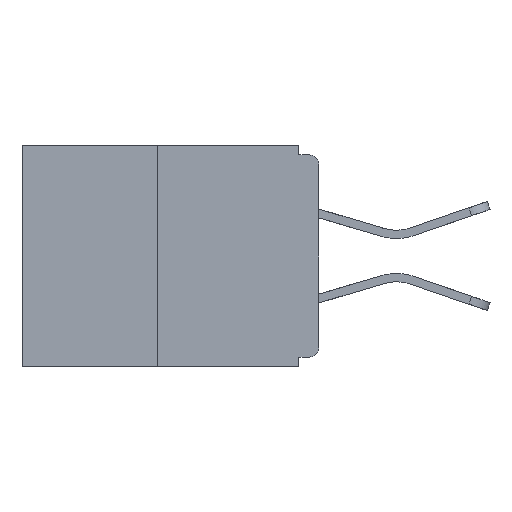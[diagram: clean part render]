
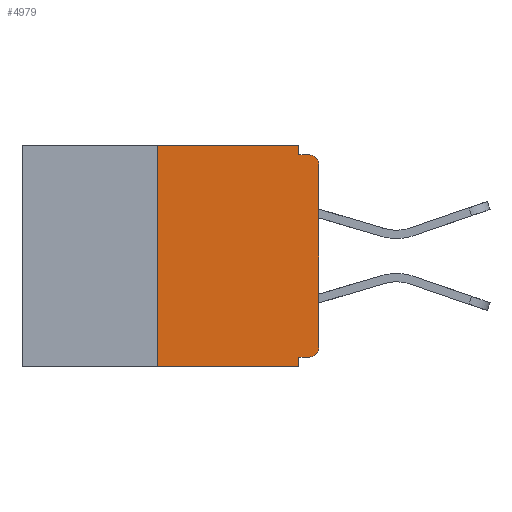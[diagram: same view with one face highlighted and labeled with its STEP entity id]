
A CAD part, left-side view. The second image highlights one B-rep face of the part: STEP entity #4979.
In plain terms, the highlighted planar face has unit normal (-1, 0, 0).
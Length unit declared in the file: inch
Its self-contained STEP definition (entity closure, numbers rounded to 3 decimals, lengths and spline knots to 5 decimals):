
#90 = AXIS2_PLACEMENT_3D ( 'NONE', #2095, #842, #13269 ) ;
#368 = VECTOR ( 'NONE', #665, 39.37008 ) ;
#665 = DIRECTION ( 'NONE',  ( 0., 0., 1. ) ) ;
#842 = DIRECTION ( 'NONE',  ( 1., 0., 0. ) ) ;
#902 = CARTESIAN_POINT ( 'NONE',  ( 0., 0.031, -0.328 ) ) ;
#1124 = VECTOR ( 'NONE', #11284, 39.37008 ) ;
#1158 = CARTESIAN_POINT ( 'NONE',  ( 0., 0.015, -0.015 ) ) ;
#1503 = LINE ( 'NONE', #16660, #368 ) ;
#1657 = EDGE_CURVE ( 'NONE', #19982, #13552, #4860, .T. ) ;
#1932 = CARTESIAN_POINT ( 'NONE',  ( 0., 0.031, -0.343 ) ) ;
#2095 = CARTESIAN_POINT ( 'NONE',  ( 0., 0.46, 0. ) ) ;
#2154 = DIRECTION ( 'NONE',  ( 0., 0., 1. ) ) ;
#2501 = CARTESIAN_POINT ( 'NONE',  ( 0., 0.46, -0.343 ) ) ;
#2604 = CARTESIAN_POINT ( 'NONE',  ( 0., 0.031, -0.343 ) ) ;
#3054 = ORIENTED_EDGE ( 'NONE', *, *, #14224, .F. ) ;
#3130 = VECTOR ( 'NONE', #14932, 39.37008 ) ;
#3685 = CIRCLE ( 'NONE', #13910, 0.015 ) ;
#3697 = EDGE_CURVE ( 'NONE', #6816, #7298, #9457, .T. ) ;
#4524 = EDGE_CURVE ( 'NONE', #9561, #6816, #18978, .T. ) ;
#4860 = LINE ( 'NONE', #2604, #21247 ) ;
#4953 = ORIENTED_EDGE ( 'NONE', *, *, #18994, .F. ) ;
#4979 = ADVANCED_FACE ( 'NONE', ( #14981 ), #9214, .F. ) ;
#5069 = DIRECTION ( 'NONE',  ( -1., 0., 0. ) ) ;
#6498 = CIRCLE ( 'NONE', #17973, 0.015 ) ;
#6816 = VERTEX_POINT ( 'NONE', #8062 ) ;
#7298 = VERTEX_POINT ( 'NONE', #1158 ) ;
#7456 = EDGE_CURVE ( 'NONE', #22584, #7298, #6498, .T. ) ;
#7811 = DIRECTION ( 'NONE',  ( 0., 0., -1. ) ) ;
#7846 = DIRECTION ( 'NONE',  ( 0., 0., -1. ) ) ;
#8062 = CARTESIAN_POINT ( 'NONE',  ( 0., 0.031, -0.015 ) ) ;
#8229 = EDGE_CURVE ( 'NONE', #9879, #22584, #1503, .T. ) ;
#8420 = EDGE_CURVE ( 'NONE', #17847, #13552, #11452, .T. ) ;
#8529 = VERTEX_POINT ( 'NONE', #22256 ) ;
#8550 = VERTEX_POINT ( 'NONE', #18922 ) ;
#8557 = CARTESIAN_POINT ( 'NONE',  ( 0., 0.015, -0.03 ) ) ;
#8724 = ORIENTED_EDGE ( 'NONE', *, *, #7456, .T. ) ;
#9059 = DIRECTION ( 'NONE',  ( 0., 0., -1. ) ) ;
#9156 = DIRECTION ( 'NONE',  ( 0., 0., -1. ) ) ;
#9214 = PLANE ( 'NONE',  #90 ) ;
#9405 = DIRECTION ( 'NONE',  ( 0., -1., 0. ) ) ;
#9457 = LINE ( 'NONE', #13211, #11985 ) ;
#9561 = VERTEX_POINT ( 'NONE', #10358 ) ;
#9618 = CARTESIAN_POINT ( 'NONE',  ( 0., 0.031, 0. ) ) ;
#9831 = ORIENTED_EDGE ( 'NONE', *, *, #12641, .T. ) ;
#9879 = VERTEX_POINT ( 'NONE', #12974 ) ;
#10358 = CARTESIAN_POINT ( 'NONE',  ( 0., 0.031, 0. ) ) ;
#10437 = ORIENTED_EDGE ( 'NONE', *, *, #8229, .T. ) ;
#10825 = VECTOR ( 'NONE', #2154, 39.37008 ) ;
#10904 = DIRECTION ( 'NONE',  ( -1., 0., 0. ) ) ;
#11284 = DIRECTION ( 'NONE',  ( 0., 1., 0. ) ) ;
#11452 = LINE ( 'NONE', #2501, #3130 ) ;
#11721 = CARTESIAN_POINT ( 'NONE',  ( 0., 0., -0.03 ) ) ;
#11985 = VECTOR ( 'NONE', #16779, 39.37008 ) ;
#12641 = EDGE_CURVE ( 'NONE', #8529, #9879, #3685, .T. ) ;
#12775 = LINE ( 'NONE', #21957, #10825 ) ;
#12927 = CARTESIAN_POINT ( 'NONE',  ( 0., 0., -0.328 ) ) ;
#12974 = CARTESIAN_POINT ( 'NONE',  ( 0., 0., -0.313 ) ) ;
#13103 = VECTOR ( 'NONE', #7811, 39.37008 ) ;
#13211 = CARTESIAN_POINT ( 'NONE',  ( 0., 0., -0.015 ) ) ;
#13269 = DIRECTION ( 'NONE',  ( 0., 0., -1. ) ) ;
#13546 = EDGE_LOOP ( 'NONE', ( #3054, #16037, #20712, #19752, #4953, #9831, #10437, #8724, #18946, #14863 ) ) ;
#13552 = VERTEX_POINT ( 'NONE', #1932 ) ;
#13674 = LINE ( 'NONE', #18593, #22311 ) ;
#13910 = AXIS2_PLACEMENT_3D ( 'NONE', #19708, #10904, #9059 ) ;
#14224 = EDGE_CURVE ( 'NONE', #8550, #9561, #13674, .T. ) ;
#14863 = ORIENTED_EDGE ( 'NONE', *, *, #4524, .F. ) ;
#14932 = DIRECTION ( 'NONE',  ( 0., -1., 0. ) ) ;
#14981 = FACE_OUTER_BOUND ( 'NONE', #13546, .T. ) ;
#16037 = ORIENTED_EDGE ( 'NONE', *, *, #18941, .F. ) ;
#16660 = CARTESIAN_POINT ( 'NONE',  ( 0., 0., 0. ) ) ;
#16779 = DIRECTION ( 'NONE',  ( 0., -1., 0. ) ) ;
#17847 = VERTEX_POINT ( 'NONE', #20184 ) ;
#17973 = AXIS2_PLACEMENT_3D ( 'NONE', #8557, #5069, #9156 ) ;
#18593 = CARTESIAN_POINT ( 'NONE',  ( 0., 0.46, 0. ) ) ;
#18922 = CARTESIAN_POINT ( 'NONE',  ( 0., 0.25, 0. ) ) ;
#18941 = EDGE_CURVE ( 'NONE', #17847, #8550, #12775, .T. ) ;
#18946 = ORIENTED_EDGE ( 'NONE', *, *, #3697, .F. ) ;
#18978 = LINE ( 'NONE', #9618, #13103 ) ;
#18994 = EDGE_CURVE ( 'NONE', #8529, #19982, #22254, .T. ) ;
#19708 = CARTESIAN_POINT ( 'NONE',  ( 0., 0.015, -0.313 ) ) ;
#19752 = ORIENTED_EDGE ( 'NONE', *, *, #1657, .F. ) ;
#19982 = VERTEX_POINT ( 'NONE', #902 ) ;
#20184 = CARTESIAN_POINT ( 'NONE',  ( 0., 0.25, -0.343 ) ) ;
#20712 = ORIENTED_EDGE ( 'NONE', *, *, #8420, .T. ) ;
#21247 = VECTOR ( 'NONE', #7846, 39.37008 ) ;
#21957 = CARTESIAN_POINT ( 'NONE',  ( 0., 0.25, 0. ) ) ;
#22254 = LINE ( 'NONE', #12927, #1124 ) ;
#22256 = CARTESIAN_POINT ( 'NONE',  ( 0., 0.015, -0.328 ) ) ;
#22311 = VECTOR ( 'NONE', #9405, 39.37008 ) ;
#22584 = VERTEX_POINT ( 'NONE', #11721 ) ;
